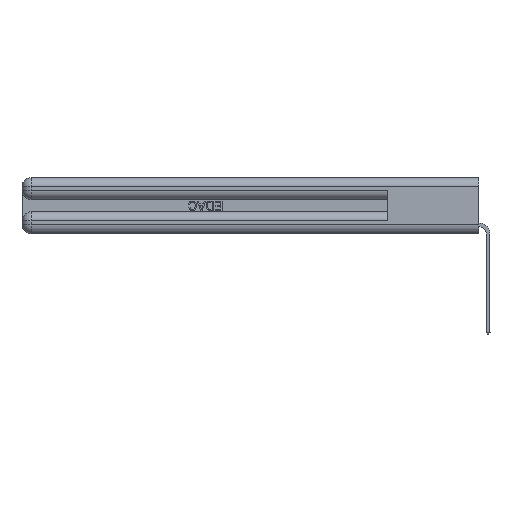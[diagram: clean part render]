
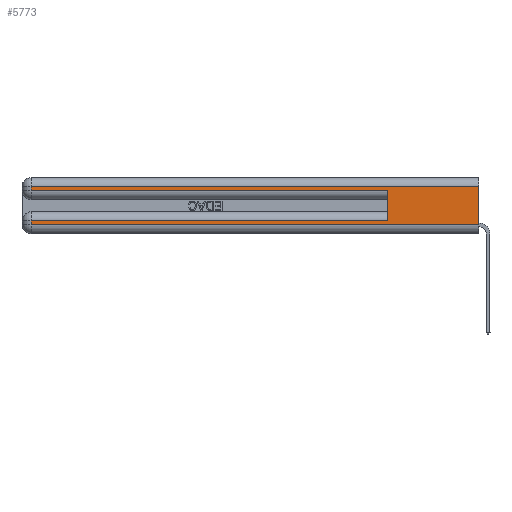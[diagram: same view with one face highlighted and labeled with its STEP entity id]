
A CAD part, left-side view. The second image highlights one B-rep face of the part: STEP entity #5773.
In plain terms, the highlighted planar face has unit normal (-1, 0, 0).
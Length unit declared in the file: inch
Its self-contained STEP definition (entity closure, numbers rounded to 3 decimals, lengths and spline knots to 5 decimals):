
#392 = CARTESIAN_POINT ( 'NONE',  ( 0., 2.94, 0.37 ) ) ;
#443 = ORIENTED_EDGE ( 'NONE', *, *, #25950, .F. ) ;
#827 = EDGE_CURVE ( 'NONE', #939, #27848, #11077, .T. ) ;
#939 = VERTEX_POINT ( 'NONE', #13407 ) ;
#1552 = DIRECTION ( 'NONE',  ( 0., 0., 1. ) ) ;
#2696 = DIRECTION ( 'NONE',  ( 0., 0., -1. ) ) ;
#2714 = EDGE_CURVE ( 'NONE', #35452, #17550, #26272, .T. ) ;
#2800 = CARTESIAN_POINT ( 'NONE',  ( 0., 0., 0.06 ) ) ;
#2862 = ORIENTED_EDGE ( 'NONE', *, *, #2714, .F. ) ;
#3134 = VERTEX_POINT ( 'NONE', #2800 ) ;
#4027 = DIRECTION ( 'NONE',  ( 0., 1., 0. ) ) ;
#4266 = ORIENTED_EDGE ( 'NONE', *, *, #20146, .T. ) ;
#5141 = VERTEX_POINT ( 'NONE', #27978 ) ;
#5443 = CARTESIAN_POINT ( 'NONE',  ( 0., 2.94, 0.37 ) ) ;
#5773 = ADVANCED_FACE ( 'NONE', ( #8823 ), #33519, .F. ) ;
#6124 = CARTESIAN_POINT ( 'NONE',  ( 0., 0., 0.285 ) ) ;
#6296 = DIRECTION ( 'NONE',  ( 0., 0., -1. ) ) ;
#6471 = EDGE_CURVE ( 'NONE', #5141, #19500, #30326, .T. ) ;
#6686 = CARTESIAN_POINT ( 'NONE',  ( 0., 0., 0.06 ) ) ;
#7575 = CARTESIAN_POINT ( 'NONE',  ( 0., 0.6, 0.085 ) ) ;
#8152 = CARTESIAN_POINT ( 'NONE',  ( 0., 0.6, 0.285 ) ) ;
#8823 = FACE_OUTER_BOUND ( 'NONE', #35635, .T. ) ;
#8994 = LINE ( 'NONE', #6124, #28490 ) ;
#10165 = CARTESIAN_POINT ( 'NONE',  ( 0., 0., 0.085 ) ) ;
#10467 = ORIENTED_EDGE ( 'NONE', *, *, #6471, .T. ) ;
#11077 = LINE ( 'NONE', #5443, #15777 ) ;
#11376 = CARTESIAN_POINT ( 'NONE',  ( 0., 0., 0.31 ) ) ;
#12044 = VECTOR ( 'NONE', #23261, 39.37008 ) ;
#12332 = DIRECTION ( 'NONE',  ( 0., -1., 0. ) ) ;
#12334 = VERTEX_POINT ( 'NONE', #11376 ) ;
#12514 = ORIENTED_EDGE ( 'NONE', *, *, #19459, .T. ) ;
#12831 = CARTESIAN_POINT ( 'NONE',  ( 0., 2.94, 0.06 ) ) ;
#12908 = LINE ( 'NONE', #34687, #32564 ) ;
#13407 = CARTESIAN_POINT ( 'NONE',  ( 0., 2.94, 0.085 ) ) ;
#13416 = LINE ( 'NONE', #10165, #15441 ) ;
#14500 = LINE ( 'NONE', #6686, #16383 ) ;
#15441 = VECTOR ( 'NONE', #18478, 39.37008 ) ;
#15777 = VECTOR ( 'NONE', #2696, 39.37008 ) ;
#16383 = VECTOR ( 'NONE', #12332, 39.37008 ) ;
#17550 = VERTEX_POINT ( 'NONE', #8152 ) ;
#18478 = DIRECTION ( 'NONE',  ( 0., 1., 0. ) ) ;
#18734 = EDGE_CURVE ( 'NONE', #35452, #939, #13416, .T. ) ;
#19459 = EDGE_CURVE ( 'NONE', #19500, #17550, #8994, .T. ) ;
#19500 = VERTEX_POINT ( 'NONE', #20024 ) ;
#19523 = ORIENTED_EDGE ( 'NONE', *, *, #827, .T. ) ;
#20024 = CARTESIAN_POINT ( 'NONE',  ( 0., 2.94, 0.285 ) ) ;
#20146 = EDGE_CURVE ( 'NONE', #27848, #3134, #14500, .T. ) ;
#21095 = CARTESIAN_POINT ( 'NONE',  ( 0., 0., 0.37 ) ) ;
#22610 = EDGE_CURVE ( 'NONE', #12334, #5141, #12908, .T. ) ;
#23261 = DIRECTION ( 'NONE',  ( 0., 0., -1. ) ) ;
#23399 = CARTESIAN_POINT ( 'NONE',  ( 0., 0.6, 0.145 ) ) ;
#25255 = DIRECTION ( 'NONE',  ( 0., -1., 0. ) ) ;
#25950 = EDGE_CURVE ( 'NONE', #12334, #3134, #29039, .T. ) ;
#26272 = LINE ( 'NONE', #23399, #29102 ) ;
#27555 = ORIENTED_EDGE ( 'NONE', *, *, #18734, .T. ) ;
#27808 = DIRECTION ( 'NONE',  ( 0., 0., -1. ) ) ;
#27848 = VERTEX_POINT ( 'NONE', #12831 ) ;
#27978 = CARTESIAN_POINT ( 'NONE',  ( 0., 2.94, 0.31 ) ) ;
#28490 = VECTOR ( 'NONE', #25255, 39.37008 ) ;
#28658 = AXIS2_PLACEMENT_3D ( 'NONE', #34217, #31334, #6296 ) ;
#28944 = ORIENTED_EDGE ( 'NONE', *, *, #22610, .T. ) ;
#29039 = LINE ( 'NONE', #21095, #12044 ) ;
#29102 = VECTOR ( 'NONE', #1552, 39.37008 ) ;
#30326 = LINE ( 'NONE', #392, #30966 ) ;
#30966 = VECTOR ( 'NONE', #27808, 39.37008 ) ;
#31334 = DIRECTION ( 'NONE',  ( 1., 0., 0. ) ) ;
#32564 = VECTOR ( 'NONE', #4027, 39.37008 ) ;
#33519 = PLANE ( 'NONE',  #28658 ) ;
#34217 = CARTESIAN_POINT ( 'NONE',  ( 0., 0., 0.37 ) ) ;
#34687 = CARTESIAN_POINT ( 'NONE',  ( 0., 0., 0.31 ) ) ;
#35452 = VERTEX_POINT ( 'NONE', #7575 ) ;
#35635 = EDGE_LOOP ( 'NONE', ( #443, #28944, #10467, #12514, #2862, #27555, #19523, #4266 ) ) ;
